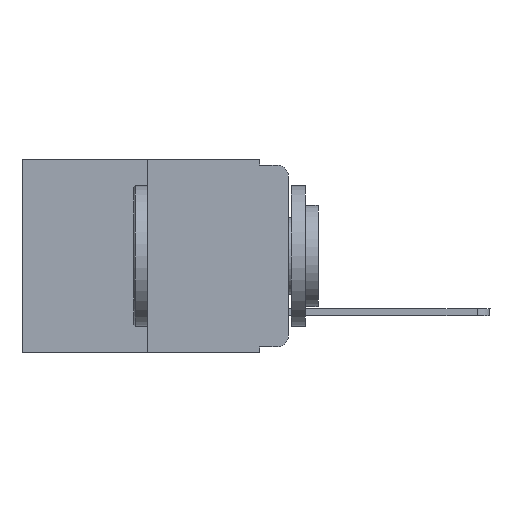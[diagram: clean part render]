
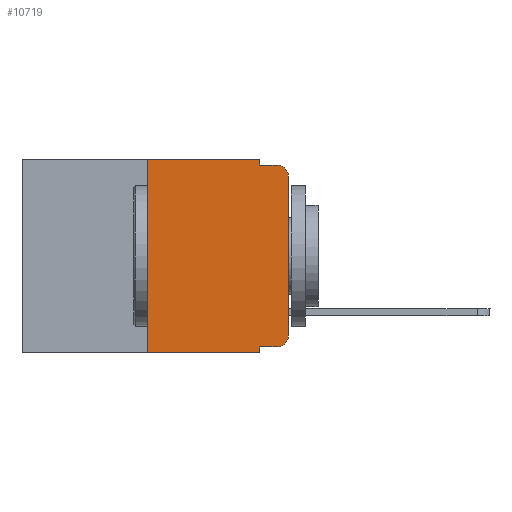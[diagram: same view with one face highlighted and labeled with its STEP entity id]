
A CAD part, left-side view. The second image highlights one B-rep face of the part: STEP entity #10719.
In plain terms, the highlighted planar face has unit normal (-1, 0, 0).
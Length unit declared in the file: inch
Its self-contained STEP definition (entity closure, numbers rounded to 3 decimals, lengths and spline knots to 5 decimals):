
#1 = VECTOR ( 'NONE', #5153, 39.37008 ) ;
#25 = VECTOR ( 'NONE', #5370, 39.37008 ) ;
#65 = CARTESIAN_POINT ( 'NONE',  ( 0., 0.473, -0.343 ) ) ;
#157 = CARTESIAN_POINT ( 'NONE',  ( 0., 0.051, 0. ) ) ;
#164 = CARTESIAN_POINT ( 'NONE',  ( 0., 0.051, -0.343 ) ) ;
#285 = LINE ( 'NONE', #2898, #2149 ) ;
#407 = ORIENTED_EDGE ( 'NONE', *, *, #1968, .F. ) ;
#492 = VECTOR ( 'NONE', #1996, 39.37008 ) ;
#857 = EDGE_CURVE ( 'NONE', #3082, #3561, #10182, .T. ) ;
#868 = EDGE_CURVE ( 'NONE', #1805, #6353, #5836, .T. ) ;
#1018 = CARTESIAN_POINT ( 'NONE',  ( 0., 0.051, -0.01 ) ) ;
#1199 = VECTOR ( 'NONE', #1954, 39.37008 ) ;
#1202 = CARTESIAN_POINT ( 'NONE',  ( 0., 0.051, -0.333 ) ) ;
#1354 = CARTESIAN_POINT ( 'NONE',  ( 0., 0.02, -0.01 ) ) ;
#1450 = CARTESIAN_POINT ( 'NONE',  ( 0., 0.25, -0.343 ) ) ;
#1590 = LINE ( 'NONE', #65, #3794 ) ;
#1591 = CARTESIAN_POINT ( 'NONE',  ( 0., 0.473, 0. ) ) ;
#1793 = VERTEX_POINT ( 'NONE', #4189 ) ;
#1805 = VERTEX_POINT ( 'NONE', #4249 ) ;
#1828 = DIRECTION ( 'NONE',  ( 0., 0., 1. ) ) ;
#1954 = DIRECTION ( 'NONE',  ( 0., -1., 0. ) ) ;
#1968 = EDGE_CURVE ( 'NONE', #1793, #6353, #7244, .T. ) ;
#1971 = DIRECTION ( 'NONE',  ( 1., 0., 0. ) ) ;
#1996 = DIRECTION ( 'NONE',  ( 0., -1., 0. ) ) ;
#2119 = ORIENTED_EDGE ( 'NONE', *, *, #7422, .T. ) ;
#2149 = VECTOR ( 'NONE', #5298, 39.37008 ) ;
#2151 = ORIENTED_EDGE ( 'NONE', *, *, #857, .F. ) ;
#2271 = CARTESIAN_POINT ( 'NONE',  ( 0., 0.02, -0.333 ) ) ;
#2435 = DIRECTION ( 'NONE',  ( 0., 0., -1. ) ) ;
#2445 = VERTEX_POINT ( 'NONE', #164 ) ;
#2555 = AXIS2_PLACEMENT_3D ( 'NONE', #10748, #1971, #5416 ) ;
#2604 = EDGE_CURVE ( 'NONE', #6244, #3182, #8188, .T. ) ;
#2625 = CARTESIAN_POINT ( 'NONE',  ( 0., 0., -0.313 ) ) ;
#2874 = FACE_OUTER_BOUND ( 'NONE', #8114, .T. ) ;
#2898 = CARTESIAN_POINT ( 'NONE',  ( 0., 0., 0. ) ) ;
#3082 = VERTEX_POINT ( 'NONE', #3208 ) ;
#3182 = VERTEX_POINT ( 'NONE', #2625 ) ;
#3208 = CARTESIAN_POINT ( 'NONE',  ( 0., 0.25, 0. ) ) ;
#3262 = ORIENTED_EDGE ( 'NONE', *, *, #10696, .F. ) ;
#3286 = EDGE_CURVE ( 'NONE', #10615, #6244, #9914, .T. ) ;
#3300 = CARTESIAN_POINT ( 'NONE',  ( 0., 0.02, -0.03 ) ) ;
#3520 = DIRECTION ( 'NONE',  ( 0., -1., 0. ) ) ;
#3561 = VERTEX_POINT ( 'NONE', #5330 ) ;
#3568 = AXIS2_PLACEMENT_3D ( 'NONE', #10354, #6876, #5825 ) ;
#3794 = VECTOR ( 'NONE', #3520, 39.37008 ) ;
#4007 = VECTOR ( 'NONE', #1828, 39.37008 ) ;
#4023 = LINE ( 'NONE', #4952, #7727 ) ;
#4189 = CARTESIAN_POINT ( 'NONE',  ( 0., 0.051, -0.01 ) ) ;
#4238 = EDGE_CURVE ( 'NONE', #3561, #1793, #4023, .T. ) ;
#4249 = CARTESIAN_POINT ( 'NONE',  ( 0., 0., -0.03 ) ) ;
#4952 = CARTESIAN_POINT ( 'NONE',  ( 0., 0.051, 0. ) ) ;
#5035 = DIRECTION ( 'NONE',  ( -1., 0., 0. ) ) ;
#5153 = DIRECTION ( 'NONE',  ( 0., -1., 0. ) ) ;
#5175 = EDGE_CURVE ( 'NONE', #7103, #2445, #1590, .T. ) ;
#5226 = ORIENTED_EDGE ( 'NONE', *, *, #868, .T. ) ;
#5298 = DIRECTION ( 'NONE',  ( 0., 0., 1. ) ) ;
#5330 = CARTESIAN_POINT ( 'NONE',  ( 0., 0.051, 0. ) ) ;
#5366 = ORIENTED_EDGE ( 'NONE', *, *, #3286, .T. ) ;
#5370 = DIRECTION ( 'NONE',  ( 0., 0., -1. ) ) ;
#5416 = DIRECTION ( 'NONE',  ( 0., 0., -1. ) ) ;
#5825 = DIRECTION ( 'NONE',  ( 0., 0., -1. ) ) ;
#5836 = CIRCLE ( 'NONE', #8244, 0.02 ) ;
#5926 = ORIENTED_EDGE ( 'NONE', *, *, #4238, .F. ) ;
#6186 = LINE ( 'NONE', #9721, #4007 ) ;
#6244 = VERTEX_POINT ( 'NONE', #2271 ) ;
#6353 = VERTEX_POINT ( 'NONE', #1354 ) ;
#6545 = ORIENTED_EDGE ( 'NONE', *, *, #10152, .F. ) ;
#6876 = DIRECTION ( 'NONE',  ( -1., 0., 0. ) ) ;
#7103 = VERTEX_POINT ( 'NONE', #1450 ) ;
#7244 = LINE ( 'NONE', #1018, #492 ) ;
#7422 = EDGE_CURVE ( 'NONE', #3182, #1805, #285, .T. ) ;
#7500 = DIRECTION ( 'NONE',  ( 0., 0., -1. ) ) ;
#7727 = VECTOR ( 'NONE', #7500, 39.37008 ) ;
#7970 = CARTESIAN_POINT ( 'NONE',  ( 0., 0.051, -0.333 ) ) ;
#8028 = PLANE ( 'NONE',  #2555 ) ;
#8114 = EDGE_LOOP ( 'NONE', ( #2119, #5226, #407, #5926, #2151, #6545, #9753, #3262, #5366, #10389 ) ) ;
#8188 = CIRCLE ( 'NONE', #3568, 0.02 ) ;
#8244 = AXIS2_PLACEMENT_3D ( 'NONE', #3300, #5035, #2435 ) ;
#9721 = CARTESIAN_POINT ( 'NONE',  ( 0., 0.25, 0. ) ) ;
#9753 = ORIENTED_EDGE ( 'NONE', *, *, #5175, .T. ) ;
#9914 = LINE ( 'NONE', #1202, #1199 ) ;
#10152 = EDGE_CURVE ( 'NONE', #7103, #3082, #6186, .T. ) ;
#10182 = LINE ( 'NONE', #1591, #1 ) ;
#10354 = CARTESIAN_POINT ( 'NONE',  ( 0., 0.02, -0.313 ) ) ;
#10389 = ORIENTED_EDGE ( 'NONE', *, *, #2604, .T. ) ;
#10615 = VERTEX_POINT ( 'NONE', #7970 ) ;
#10696 = EDGE_CURVE ( 'NONE', #10615, #2445, #10868, .T. ) ;
#10719 = ADVANCED_FACE ( 'NONE', ( #2874 ), #8028, .F. ) ;
#10748 = CARTESIAN_POINT ( 'NONE',  ( 0., 0.473, 0. ) ) ;
#10868 = LINE ( 'NONE', #157, #25 ) ;
